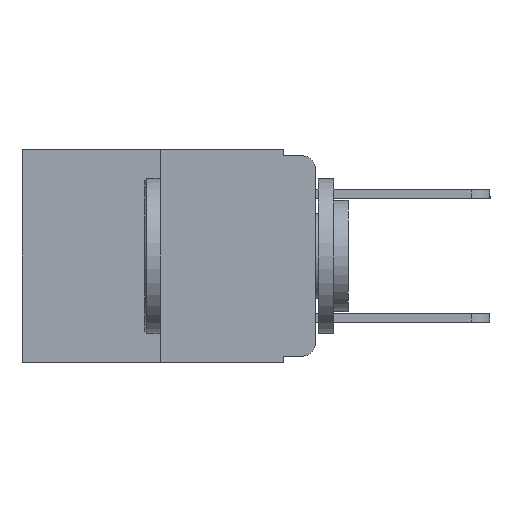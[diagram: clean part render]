
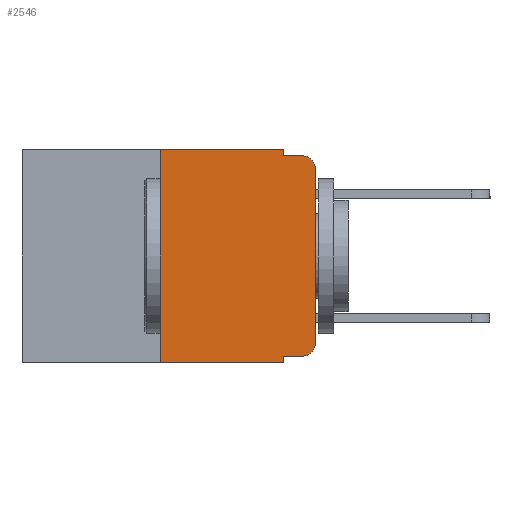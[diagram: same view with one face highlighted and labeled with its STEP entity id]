
A CAD part, left-side view. The second image highlights one B-rep face of the part: STEP entity #2546.
In plain terms, the highlighted planar face has unit normal (-1, 0, 0).
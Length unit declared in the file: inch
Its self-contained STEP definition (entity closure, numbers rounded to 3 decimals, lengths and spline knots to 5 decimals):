
#322 = CARTESIAN_POINT ( 'NONE',  ( 0., 0.051, 0. ) ) ;
#368 = AXIS2_PLACEMENT_3D ( 'NONE', #7433, #7372, #8641 ) ;
#417 = CIRCLE ( 'NONE', #1236, 0.02 ) ;
#654 = VERTEX_POINT ( 'NONE', #8319 ) ;
#821 = CARTESIAN_POINT ( 'NONE',  ( 0., 0.02, -0.333 ) ) ;
#1047 = DIRECTION ( 'NONE',  ( 0., 0., -1. ) ) ;
#1073 = CARTESIAN_POINT ( 'NONE',  ( 0., 0., 0. ) ) ;
#1104 = LINE ( 'NONE', #12374, #11292 ) ;
#1111 = ORIENTED_EDGE ( 'NONE', *, *, #2002, .T. ) ;
#1142 = EDGE_CURVE ( 'NONE', #654, #5568, #10323, .T. ) ;
#1163 = EDGE_CURVE ( 'NONE', #1956, #11289, #2456, .T. ) ;
#1236 = AXIS2_PLACEMENT_3D ( 'NONE', #7635, #5438, #6270 ) ;
#1389 = EDGE_CURVE ( 'NONE', #9527, #1956, #3862, .T. ) ;
#1390 = EDGE_CURVE ( 'NONE', #11276, #2495, #9136, .T. ) ;
#1414 = EDGE_CURVE ( 'NONE', #2495, #11289, #6900, .T. ) ;
#1496 = CARTESIAN_POINT ( 'NONE',  ( 0., 0.051, -0.01 ) ) ;
#1691 = VERTEX_POINT ( 'NONE', #12130 ) ;
#1787 = DIRECTION ( 'NONE',  ( 0., 0., 1. ) ) ;
#1880 = ORIENTED_EDGE ( 'NONE', *, *, #1960, .T. ) ;
#1956 = VERTEX_POINT ( 'NONE', #5322 ) ;
#1960 = EDGE_CURVE ( 'NONE', #3860, #11276, #417, .T. ) ;
#2002 = EDGE_CURVE ( 'NONE', #1691, #3860, #9297, .T. ) ;
#2015 = CARTESIAN_POINT ( 'NONE',  ( 0., 0.02, -0.01 ) ) ;
#2127 = CARTESIAN_POINT ( 'NONE',  ( 0., 0.473, 0. ) ) ;
#2335 = AXIS2_PLACEMENT_3D ( 'NONE', #2127, #10451, #11172 ) ;
#2382 = CARTESIAN_POINT ( 'NONE',  ( 0., 0.25, 0. ) ) ;
#2456 = LINE ( 'NONE', #1496, #4791 ) ;
#2495 = VERTEX_POINT ( 'NONE', #4453 ) ;
#2512 = ORIENTED_EDGE ( 'NONE', *, *, #1414, .T. ) ;
#2546 = ADVANCED_FACE ( 'NONE', ( #10917 ), #10289, .F. ) ;
#2572 = VECTOR ( 'NONE', #10477, 39.37008 ) ;
#2886 = ORIENTED_EDGE ( 'NONE', *, *, #1163, .F. ) ;
#3251 = ORIENTED_EDGE ( 'NONE', *, *, #3527, .F. ) ;
#3344 = CARTESIAN_POINT ( 'NONE',  ( 0., 0.051, 0. ) ) ;
#3473 = ORIENTED_EDGE ( 'NONE', *, *, #1389, .F. ) ;
#3527 = EDGE_CURVE ( 'NONE', #1691, #11846, #8426, .T. ) ;
#3841 = ORIENTED_EDGE ( 'NONE', *, *, #1390, .T. ) ;
#3860 = VERTEX_POINT ( 'NONE', #821 ) ;
#3862 = LINE ( 'NONE', #322, #9412 ) ;
#4255 = DIRECTION ( 'NONE',  ( 0., -1., 0. ) ) ;
#4424 = ORIENTED_EDGE ( 'NONE', *, *, #7699, .F. ) ;
#4453 = CARTESIAN_POINT ( 'NONE',  ( 0., 0., -0.03 ) ) ;
#4491 = DIRECTION ( 'NONE',  ( 0., -1., 0. ) ) ;
#4791 = VECTOR ( 'NONE', #4491, 39.37008 ) ;
#5026 = EDGE_LOOP ( 'NONE', ( #3841, #2512, #2886, #3473, #4424, #5327, #6410, #3251, #1111, #1880 ) ) ;
#5137 = DIRECTION ( 'NONE',  ( 0., 0., 1. ) ) ;
#5170 = VECTOR ( 'NONE', #1787, 39.37008 ) ;
#5322 = CARTESIAN_POINT ( 'NONE',  ( 0., 0.051, -0.01 ) ) ;
#5327 = ORIENTED_EDGE ( 'NONE', *, *, #1142, .F. ) ;
#5438 = DIRECTION ( 'NONE',  ( -1., 0., 0. ) ) ;
#5568 = VERTEX_POINT ( 'NONE', #11100 ) ;
#6270 = DIRECTION ( 'NONE',  ( 0., 0., -1. ) ) ;
#6410 = ORIENTED_EDGE ( 'NONE', *, *, #8135, .T. ) ;
#6563 = VECTOR ( 'NONE', #5137, 39.37008 ) ;
#6759 = CARTESIAN_POINT ( 'NONE',  ( 0., 0.473, 0. ) ) ;
#6900 = CIRCLE ( 'NONE', #368, 0.02 ) ;
#7372 = DIRECTION ( 'NONE',  ( -1., 0., 0. ) ) ;
#7433 = CARTESIAN_POINT ( 'NONE',  ( 0., 0.02, -0.03 ) ) ;
#7635 = CARTESIAN_POINT ( 'NONE',  ( 0., 0.02, -0.313 ) ) ;
#7699 = EDGE_CURVE ( 'NONE', #5568, #9527, #11424, .T. ) ;
#8135 = EDGE_CURVE ( 'NONE', #654, #11846, #1104, .T. ) ;
#8319 = CARTESIAN_POINT ( 'NONE',  ( 0., 0.25, -0.343 ) ) ;
#8426 = LINE ( 'NONE', #10979, #2572 ) ;
#8641 = DIRECTION ( 'NONE',  ( 0., 0., -1. ) ) ;
#9136 = LINE ( 'NONE', #1073, #6563 ) ;
#9297 = LINE ( 'NONE', #10847, #10934 ) ;
#9336 = VECTOR ( 'NONE', #11151, 39.37008 ) ;
#9412 = VECTOR ( 'NONE', #1047, 39.37008 ) ;
#9527 = VERTEX_POINT ( 'NONE', #3344 ) ;
#10289 = PLANE ( 'NONE',  #2335 ) ;
#10315 = CARTESIAN_POINT ( 'NONE',  ( 0., 0., -0.313 ) ) ;
#10323 = LINE ( 'NONE', #2382, #5170 ) ;
#10374 = DIRECTION ( 'NONE',  ( 0., -1., 0. ) ) ;
#10451 = DIRECTION ( 'NONE',  ( 1., 0., 0. ) ) ;
#10477 = DIRECTION ( 'NONE',  ( 0., 0., -1. ) ) ;
#10847 = CARTESIAN_POINT ( 'NONE',  ( 0., 0.051, -0.333 ) ) ;
#10917 = FACE_OUTER_BOUND ( 'NONE', #5026, .T. ) ;
#10934 = VECTOR ( 'NONE', #10374, 39.37008 ) ;
#10979 = CARTESIAN_POINT ( 'NONE',  ( 0., 0.051, 0. ) ) ;
#11100 = CARTESIAN_POINT ( 'NONE',  ( 0., 0.25, 0. ) ) ;
#11151 = DIRECTION ( 'NONE',  ( 0., -1., 0. ) ) ;
#11172 = DIRECTION ( 'NONE',  ( 0., 0., -1. ) ) ;
#11276 = VERTEX_POINT ( 'NONE', #10315 ) ;
#11289 = VERTEX_POINT ( 'NONE', #2015 ) ;
#11292 = VECTOR ( 'NONE', #4255, 39.37008 ) ;
#11424 = LINE ( 'NONE', #6759, #9336 ) ;
#11846 = VERTEX_POINT ( 'NONE', #12678 ) ;
#12130 = CARTESIAN_POINT ( 'NONE',  ( 0., 0.051, -0.333 ) ) ;
#12374 = CARTESIAN_POINT ( 'NONE',  ( 0., 0.473, -0.343 ) ) ;
#12678 = CARTESIAN_POINT ( 'NONE',  ( 0., 0.051, -0.343 ) ) ;
